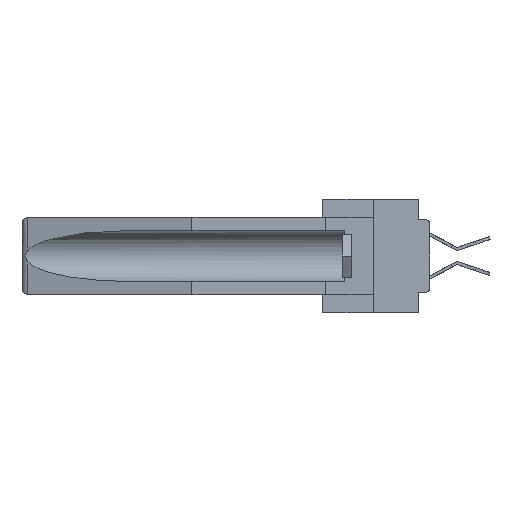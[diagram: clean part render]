
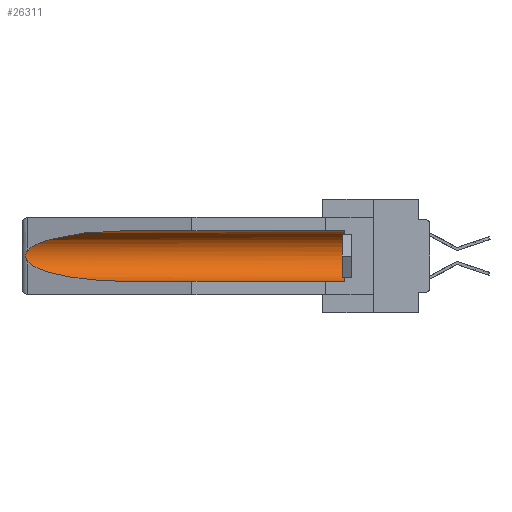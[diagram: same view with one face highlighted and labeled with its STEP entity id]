
A CAD part, left-side view. The second image highlights one B-rep face of the part: STEP entity #26311.
In plain terms, the highlighted cylindrical face has radius 2.857 mm (diameter 5.715 mm), a partial arc.
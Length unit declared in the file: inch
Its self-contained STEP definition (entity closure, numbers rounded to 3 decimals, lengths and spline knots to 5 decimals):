
#745 = ORIENTED_EDGE ( 'NONE', *, *, #18535, .T. ) ;
#1122 = EDGE_CURVE ( 'NONE', #4274, #25793, #9552, .T. ) ;
#1685 = ORIENTED_EDGE ( 'NONE', *, *, #6692, .T. ) ;
#1797 = CARTESIAN_POINT ( 'NONE',  ( 0.26654, 1.53092, -0.15636 ) ) ;
#1881 = CARTESIAN_POINT ( 'NONE',  ( 0.25451, 1.48313, -0.24835 ) ) ;
#2767 = CARTESIAN_POINT ( 'NONE',  ( 0.26537, 1.52718, -0.19328 ) ) ;
#2873 = VERTEX_POINT ( 'NONE', #3754 ) ;
#2992 = AXIS2_PLACEMENT_3D ( 'NONE', #35344, #23249, #9523 ) ;
#3239 = EDGE_CURVE ( 'NONE', #2873, #4274, #4265, .T. ) ;
#3754 = CARTESIAN_POINT ( 'NONE',  ( 0.26537, 1.52718, -0.14972 ) ) ;
#3941 = DIRECTION ( 'NONE',  ( 0., 1., 0. ) ) ;
#4158 = CARTESIAN_POINT ( 'NONE',  ( 0.26655, 1.53094, -0.18657 ) ) ;
#4265 = B_SPLINE_CURVE_WITH_KNOTS ( 'NONE', 3,
 ( #26328, #18328, #1797, #15694, #20888, #18070, #29112, #4158, #6916, #7290 ),
 .UNSPECIFIED., .F., .F.,
 ( 4, 2, 2, 2, 4 ),
 ( 0., 0.00029, 0.00058, 0.00087, 0.00117 ),
 .UNSPECIFIED. ) ;
#4274 = VERTEX_POINT ( 'NONE', #2767 ) ;
#4979 = CARTESIAN_POINT ( 'NONE',  ( 0.155, 0.126, -0.284 ) ) ;
#6316 = CARTESIAN_POINT ( 'NONE',  ( 0.155, -0.30754, -0.059 ) ) ;
#6476 =( BOUNDED_CURVE ( )  B_SPLINE_CURVE ( 3, ( #33303, #25092, #30644, #30532 ),
 .UNSPECIFIED., .F., .F. ) 
 B_SPLINE_CURVE_WITH_KNOTS ( ( 4, 4 ),
 ( 4.71239, 6.08839 ),
 .UNSPECIFIED. ) 
 CURVE ( )  GEOMETRIC_REPRESENTATION_ITEM ( )  RATIONAL_B_SPLINE_CURVE ( ( 1., 0.848, 0.848, 1. ) ) 
 REPRESENTATION_ITEM ( '' )  );
#6692 = EDGE_CURVE ( 'NONE', #12660, #27573, #7555, .T. ) ;
#6916 = CARTESIAN_POINT ( 'NONE',  ( 0.26597, 1.5296, -0.19026 ) ) ;
#7290 = CARTESIAN_POINT ( 'NONE',  ( 0.26537, 1.52718, -0.19328 ) ) ;
#7363 = CARTESIAN_POINT ( 'NONE',  ( 0.155, 0.126, -0.1715 ) ) ;
#7555 = LINE ( 'NONE', #6316, #14391 ) ;
#9362 = AXIS2_PLACEMENT_3D ( 'NONE', #7363, #20842, #26662 ) ;
#9523 = DIRECTION ( 'NONE',  ( 0., 0., 1. ) ) ;
#9552 =( BOUNDED_CURVE ( )  B_SPLINE_CURVE ( 3, ( #29292, #1881, #10124, #29418 ),
 .UNSPECIFIED., .F., .F. ) 
 B_SPLINE_CURVE_WITH_KNOTS ( ( 4, 4 ),
 ( 0.1948, 1.5708 ),
 .UNSPECIFIED. ) 
 CURVE ( )  GEOMETRIC_REPRESENTATION_ITEM ( )  RATIONAL_B_SPLINE_CURVE ( ( 1., 0.848, 0.848, 1. ) ) 
 REPRESENTATION_ITEM ( '' )  );
#10124 = CARTESIAN_POINT ( 'NONE',  ( 0.21114, 1.30732, -0.284 ) ) ;
#12464 = VERTEX_POINT ( 'NONE', #4979 ) ;
#12660 = VERTEX_POINT ( 'NONE', #14667 ) ;
#13379 = EDGE_CURVE ( 'NONE', #12464, #12660, #22977, .T. ) ;
#14391 = VECTOR ( 'NONE', #17332, 39.37008 ) ;
#14667 = CARTESIAN_POINT ( 'NONE',  ( 0.155, 0.126, -0.059 ) ) ;
#15694 = CARTESIAN_POINT ( 'NONE',  ( 0.2673, 1.5327, -0.16383 ) ) ;
#16016 = ORIENTED_EDGE ( 'NONE', *, *, #3239, .T. ) ;
#16515 = LINE ( 'NONE', #20783, #22985 ) ;
#16983 = CYLINDRICAL_SURFACE ( 'NONE', #2992, 0.1125 ) ;
#17332 = DIRECTION ( 'NONE',  ( 0., 1., 0. ) ) ;
#18070 = CARTESIAN_POINT ( 'NONE',  ( 0.2675, 1.53308, -0.17534 ) ) ;
#18328 = CARTESIAN_POINT ( 'NONE',  ( 0.26597, 1.52961, -0.15275 ) ) ;
#18535 = EDGE_CURVE ( 'NONE', #27573, #2873, #6476, .T. ) ;
#20783 = CARTESIAN_POINT ( 'NONE',  ( 0.155, -0.30754, -0.284 ) ) ;
#20842 = DIRECTION ( 'NONE',  ( 0., -1., 0. ) ) ;
#20888 = CARTESIAN_POINT ( 'NONE',  ( 0.2675, 1.53308, -0.16763 ) ) ;
#21913 = ORIENTED_EDGE ( 'NONE', *, *, #13379, .T. ) ;
#22977 = CIRCLE ( 'NONE', #9362, 0.1125 ) ;
#22985 = VECTOR ( 'NONE', #3941, 39.37008 ) ;
#23206 = ORIENTED_EDGE ( 'NONE', *, *, #1122, .T. ) ;
#23249 = DIRECTION ( 'NONE',  ( 0., 1., 0. ) ) ;
#24500 = CARTESIAN_POINT ( 'NONE',  ( 0.155, 1.07973, -0.284 ) ) ;
#24761 = FACE_OUTER_BOUND ( 'NONE', #28038, .T. ) ;
#25092 = CARTESIAN_POINT ( 'NONE',  ( 0.21114, 1.30732, -0.059 ) ) ;
#25793 = VERTEX_POINT ( 'NONE', #24500 ) ;
#26311 = ADVANCED_FACE ( 'NONE', ( #24761 ), #16983, .F. ) ;
#26328 = CARTESIAN_POINT ( 'NONE',  ( 0.26537, 1.52718, -0.14972 ) ) ;
#26662 = DIRECTION ( 'NONE',  ( 0., 0., 1. ) ) ;
#27573 = VERTEX_POINT ( 'NONE', #35389 ) ;
#28038 = EDGE_LOOP ( 'NONE', ( #745, #16016, #23206, #31662, #21913, #1685 ) ) ;
#29112 = CARTESIAN_POINT ( 'NONE',  ( 0.2673, 1.53269, -0.17917 ) ) ;
#29292 = CARTESIAN_POINT ( 'NONE',  ( 0.26537, 1.52718, -0.19328 ) ) ;
#29418 = CARTESIAN_POINT ( 'NONE',  ( 0.155, 1.07973, -0.284 ) ) ;
#29926 = EDGE_CURVE ( 'NONE', #12464, #25793, #16515, .T. ) ;
#30532 = CARTESIAN_POINT ( 'NONE',  ( 0.26537, 1.52718, -0.14972 ) ) ;
#30644 = CARTESIAN_POINT ( 'NONE',  ( 0.25451, 1.48313, -0.09465 ) ) ;
#31662 = ORIENTED_EDGE ( 'NONE', *, *, #29926, .F. ) ;
#33303 = CARTESIAN_POINT ( 'NONE',  ( 0.155, 1.07973, -0.059 ) ) ;
#35344 = CARTESIAN_POINT ( 'NONE',  ( 0.155, -0.30754, -0.1715 ) ) ;
#35389 = CARTESIAN_POINT ( 'NONE',  ( 0.155, 1.07973, -0.059 ) ) ;
